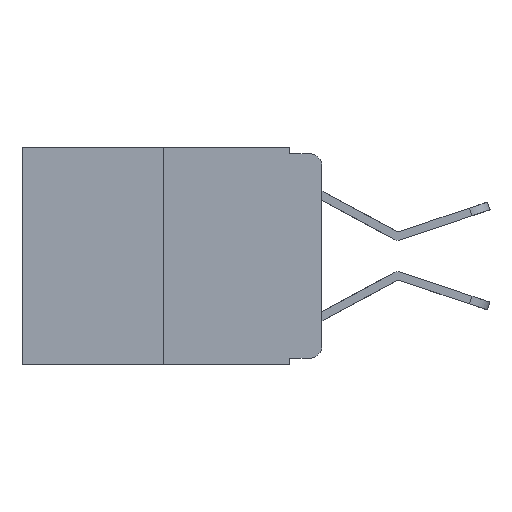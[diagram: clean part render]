
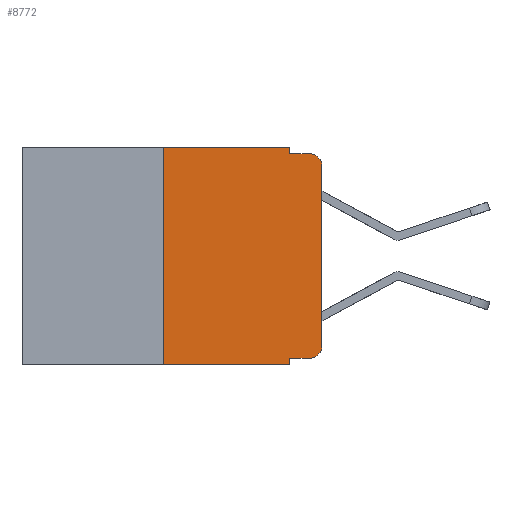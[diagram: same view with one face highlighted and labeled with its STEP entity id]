
A CAD part, left-side view. The second image highlights one B-rep face of the part: STEP entity #8772.
In plain terms, the highlighted planar face has unit normal (-1, 0, 0).
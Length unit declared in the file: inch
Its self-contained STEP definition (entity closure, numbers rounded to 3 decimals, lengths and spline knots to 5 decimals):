
#685 = ORIENTED_EDGE ( 'NONE', *, *, #19815, .F. ) ;
#1599 = CARTESIAN_POINT ( 'NONE',  ( 0., 0.051, 0. ) ) ;
#1640 = CARTESIAN_POINT ( 'NONE',  ( 0., 0.051, -0.333 ) ) ;
#1993 = VECTOR ( 'NONE', #20443, 39.37008 ) ;
#2467 = VERTEX_POINT ( 'NONE', #16932 ) ;
#2644 = ORIENTED_EDGE ( 'NONE', *, *, #16538, .F. ) ;
#3206 = ORIENTED_EDGE ( 'NONE', *, *, #18731, .F. ) ;
#3386 = DIRECTION ( 'NONE',  ( 0., 0., -1. ) ) ;
#3443 = LINE ( 'NONE', #21696, #7463 ) ;
#3487 = DIRECTION ( 'NONE',  ( 0., -1., 0. ) ) ;
#4080 = CARTESIAN_POINT ( 'NONE',  ( 0., 0.25, -0.343 ) ) ;
#4116 = VERTEX_POINT ( 'NONE', #7731 ) ;
#4237 = CARTESIAN_POINT ( 'NONE',  ( 0., 0.02, -0.03 ) ) ;
#4278 = CARTESIAN_POINT ( 'NONE',  ( 0., 0.473, 0. ) ) ;
#4520 = VERTEX_POINT ( 'NONE', #10833 ) ;
#4965 = EDGE_CURVE ( 'NONE', #13300, #15920, #9773, .T. ) ;
#5099 = EDGE_CURVE ( 'NONE', #6673, #18063, #11071, .T. ) ;
#5927 = ORIENTED_EDGE ( 'NONE', *, *, #6127, .T. ) ;
#5940 = PLANE ( 'NONE',  #19957 ) ;
#5972 = DIRECTION ( 'NONE',  ( 0., 0., -1. ) ) ;
#6007 = DIRECTION ( 'NONE',  ( 0., 0., -1. ) ) ;
#6127 = EDGE_CURVE ( 'NONE', #11795, #2467, #21588, .T. ) ;
#6552 = EDGE_CURVE ( 'NONE', #4116, #9631, #18781, .T. ) ;
#6673 = VERTEX_POINT ( 'NONE', #4080 ) ;
#7000 = DIRECTION ( 'NONE',  ( 0., -1., 0. ) ) ;
#7129 = EDGE_LOOP ( 'NONE', ( #18349, #14516, #15032, #2644, #16054, #3206, #12224, #685, #5927, #14775 ) ) ;
#7160 = LINE ( 'NONE', #8434, #19775 ) ;
#7382 = VECTOR ( 'NONE', #9182, 39.37008 ) ;
#7463 = VECTOR ( 'NONE', #3487, 39.37008 ) ;
#7731 = CARTESIAN_POINT ( 'NONE',  ( 0., 0., -0.313 ) ) ;
#8371 = EDGE_CURVE ( 'NONE', #2467, #4116, #8911, .T. ) ;
#8375 = CARTESIAN_POINT ( 'NONE',  ( 0., 0.02, -0.313 ) ) ;
#8434 = CARTESIAN_POINT ( 'NONE',  ( 0., 0.051, 0. ) ) ;
#8772 = ADVANCED_FACE ( 'NONE', ( #9423 ), #5940, .F. ) ;
#8911 = CIRCLE ( 'NONE', #11631, 0.02 ) ;
#9182 = DIRECTION ( 'NONE',  ( 0., 0., 1. ) ) ;
#9407 = CIRCLE ( 'NONE', #11785, 0.02 ) ;
#9423 = FACE_OUTER_BOUND ( 'NONE', #7129, .T. ) ;
#9631 = VERTEX_POINT ( 'NONE', #11863 ) ;
#9773 = LINE ( 'NONE', #15263, #21291 ) ;
#9945 = EDGE_CURVE ( 'NONE', #9631, #4520, #9407, .T. ) ;
#10090 = DIRECTION ( 'NONE',  ( 0., 0., -1. ) ) ;
#10148 = DIRECTION ( 'NONE',  ( 0., 0., -1. ) ) ;
#10833 = CARTESIAN_POINT ( 'NONE',  ( 0., 0.02, -0.01 ) ) ;
#11007 = LINE ( 'NONE', #1599, #16403 ) ;
#11071 = LINE ( 'NONE', #18823, #1993 ) ;
#11631 = AXIS2_PLACEMENT_3D ( 'NONE', #8375, #19880, #10090 ) ;
#11785 = AXIS2_PLACEMENT_3D ( 'NONE', #4237, #15921, #5972 ) ;
#11795 = VERTEX_POINT ( 'NONE', #1640 ) ;
#11863 = CARTESIAN_POINT ( 'NONE',  ( 0., 0., -0.03 ) ) ;
#12224 = ORIENTED_EDGE ( 'NONE', *, *, #5099, .T. ) ;
#12921 = VECTOR ( 'NONE', #16083, 39.37008 ) ;
#13300 = VERTEX_POINT ( 'NONE', #14458 ) ;
#13933 = VECTOR ( 'NONE', #20328, 39.37008 ) ;
#14441 = CARTESIAN_POINT ( 'NONE',  ( 0., 0.051, -0.333 ) ) ;
#14458 = CARTESIAN_POINT ( 'NONE',  ( 0., 0.25, 0. ) ) ;
#14516 = ORIENTED_EDGE ( 'NONE', *, *, #9945, .T. ) ;
#14775 = ORIENTED_EDGE ( 'NONE', *, *, #8371, .T. ) ;
#15032 = ORIENTED_EDGE ( 'NONE', *, *, #15459, .F. ) ;
#15263 = CARTESIAN_POINT ( 'NONE',  ( 0., 0.473, 0. ) ) ;
#15435 = CARTESIAN_POINT ( 'NONE',  ( 0., 0., 0. ) ) ;
#15459 = EDGE_CURVE ( 'NONE', #16147, #4520, #3443, .T. ) ;
#15681 = LINE ( 'NONE', #19012, #7382 ) ;
#15920 = VERTEX_POINT ( 'NONE', #17411 ) ;
#15921 = DIRECTION ( 'NONE',  ( -1., 0., 0. ) ) ;
#15964 = DIRECTION ( 'NONE',  ( 1., 0., 0. ) ) ;
#16054 = ORIENTED_EDGE ( 'NONE', *, *, #4965, .F. ) ;
#16083 = DIRECTION ( 'NONE',  ( 0., -1., 0. ) ) ;
#16147 = VERTEX_POINT ( 'NONE', #18967 ) ;
#16403 = VECTOR ( 'NONE', #3386, 39.37008 ) ;
#16538 = EDGE_CURVE ( 'NONE', #15920, #16147, #7160, .T. ) ;
#16899 = CARTESIAN_POINT ( 'NONE',  ( 0., 0.051, -0.343 ) ) ;
#16932 = CARTESIAN_POINT ( 'NONE',  ( 0., 0.02, -0.333 ) ) ;
#17411 = CARTESIAN_POINT ( 'NONE',  ( 0., 0.051, 0. ) ) ;
#18063 = VERTEX_POINT ( 'NONE', #16899 ) ;
#18349 = ORIENTED_EDGE ( 'NONE', *, *, #6552, .T. ) ;
#18731 = EDGE_CURVE ( 'NONE', #6673, #13300, #15681, .T. ) ;
#18781 = LINE ( 'NONE', #15435, #13933 ) ;
#18823 = CARTESIAN_POINT ( 'NONE',  ( 0., 0.473, -0.343 ) ) ;
#18967 = CARTESIAN_POINT ( 'NONE',  ( 0., 0.051, -0.01 ) ) ;
#19012 = CARTESIAN_POINT ( 'NONE',  ( 0., 0.25, 0. ) ) ;
#19775 = VECTOR ( 'NONE', #10148, 39.37008 ) ;
#19815 = EDGE_CURVE ( 'NONE', #11795, #18063, #11007, .T. ) ;
#19880 = DIRECTION ( 'NONE',  ( -1., 0., 0. ) ) ;
#19957 = AXIS2_PLACEMENT_3D ( 'NONE', #4278, #15964, #6007 ) ;
#20328 = DIRECTION ( 'NONE',  ( 0., 0., 1. ) ) ;
#20443 = DIRECTION ( 'NONE',  ( 0., -1., 0. ) ) ;
#21291 = VECTOR ( 'NONE', #7000, 39.37008 ) ;
#21588 = LINE ( 'NONE', #14441, #12921 ) ;
#21696 = CARTESIAN_POINT ( 'NONE',  ( 0., 0.051, -0.01 ) ) ;
